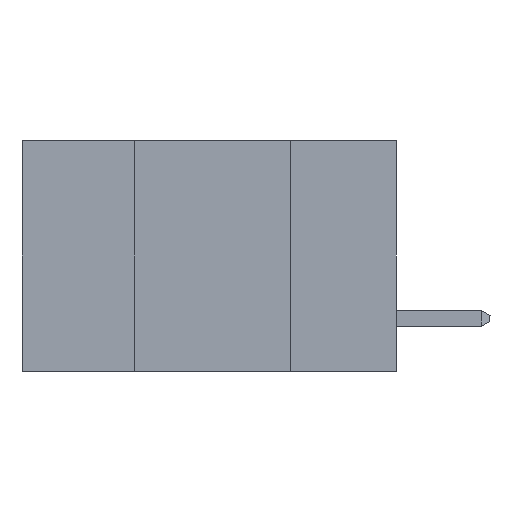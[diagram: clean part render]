
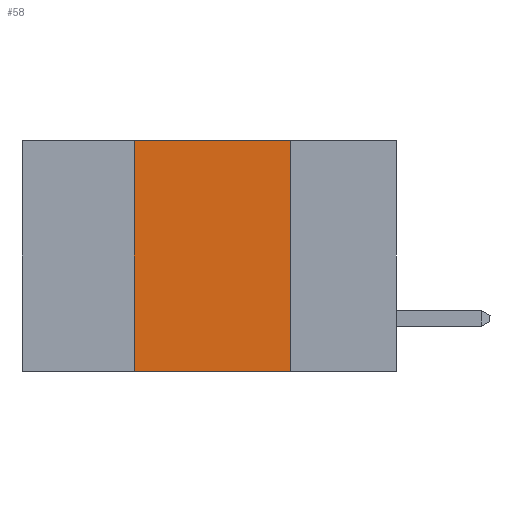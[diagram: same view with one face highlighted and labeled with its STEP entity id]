
A CAD part, left-side view. The second image highlights one B-rep face of the part: STEP entity #58.
In plain terms, the highlighted planar face has unit normal (-1, 0, 0).
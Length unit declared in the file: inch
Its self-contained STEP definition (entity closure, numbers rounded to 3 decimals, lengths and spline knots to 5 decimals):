
#58 = ADVANCED_FACE ( 'NONE', ( #14076 ), #12779, .F. ) ;
#355 = DIRECTION ( 'NONE',  ( 0., 0., -1. ) ) ;
#535 = LINE ( 'NONE', #9632, #9640 ) ;
#782 = CARTESIAN_POINT ( 'NONE',  ( 0., 0.6, 0. ) ) ;
#914 = DIRECTION ( 'NONE',  ( 0., 0., 1. ) ) ;
#3427 = VERTEX_POINT ( 'NONE', #5923 ) ;
#3694 = VERTEX_POINT ( 'NONE', #9411 ) ;
#5923 = CARTESIAN_POINT ( 'NONE',  ( 0., 0.17, 0. ) ) ;
#6785 = ORIENTED_EDGE ( 'NONE', *, *, #7174, .F. ) ;
#6977 = LINE ( 'NONE', #782, #7005 ) ;
#7005 = VECTOR ( 'NONE', #19212, 39.37008 ) ;
#7174 = EDGE_CURVE ( 'NONE', #3427, #3694, #535, .T. ) ;
#7462 = ORIENTED_EDGE ( 'NONE', *, *, #19032, .F. ) ;
#7900 = AXIS2_PLACEMENT_3D ( 'NONE', #11166, #15882, #355 ) ;
#7932 = DIRECTION ( 'NONE',  ( 0., 0., -1. ) ) ;
#8617 = VERTEX_POINT ( 'NONE', #14740 ) ;
#8689 = ORIENTED_EDGE ( 'NONE', *, *, #14738, .T. ) ;
#9189 = CARTESIAN_POINT ( 'NONE',  ( 0., 0.6, -0.37 ) ) ;
#9411 = CARTESIAN_POINT ( 'NONE',  ( 0., 0.17, -0.37 ) ) ;
#9445 = VERTEX_POINT ( 'NONE', #13649 ) ;
#9632 = CARTESIAN_POINT ( 'NONE',  ( 0., 0.17, -0.37 ) ) ;
#9640 = VECTOR ( 'NONE', #7932, 39.37008 ) ;
#9774 = EDGE_LOOP ( 'NONE', ( #6785, #7462, #16504, #8689 ) ) ;
#10453 = VECTOR ( 'NONE', #914, 39.37008 ) ;
#10770 = VECTOR ( 'NONE', #18700, 39.37008 ) ;
#11166 = CARTESIAN_POINT ( 'NONE',  ( 0., 0.6, 0. ) ) ;
#12779 = PLANE ( 'NONE',  #7900 ) ;
#13649 = CARTESIAN_POINT ( 'NONE',  ( 0., 0.42, 0. ) ) ;
#14076 = FACE_OUTER_BOUND ( 'NONE', #9774, .T. ) ;
#14485 = EDGE_CURVE ( 'NONE', #8617, #9445, #17827, .T. ) ;
#14738 = EDGE_CURVE ( 'NONE', #8617, #3694, #16812, .T. ) ;
#14740 = CARTESIAN_POINT ( 'NONE',  ( 0., 0.42, -0.37 ) ) ;
#15882 = DIRECTION ( 'NONE',  ( 1., 0., 0. ) ) ;
#16504 = ORIENTED_EDGE ( 'NONE', *, *, #14485, .F. ) ;
#16812 = LINE ( 'NONE', #9189, #10770 ) ;
#17827 = LINE ( 'NONE', #18939, #10453 ) ;
#18700 = DIRECTION ( 'NONE',  ( 0., -1., 0. ) ) ;
#18939 = CARTESIAN_POINT ( 'NONE',  ( 0., 0.42, -0.37 ) ) ;
#19032 = EDGE_CURVE ( 'NONE', #9445, #3427, #6977, .T. ) ;
#19212 = DIRECTION ( 'NONE',  ( 0., -1., 0. ) ) ;
